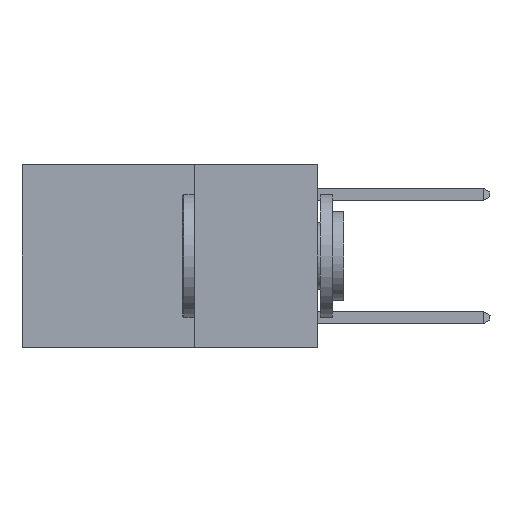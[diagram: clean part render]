
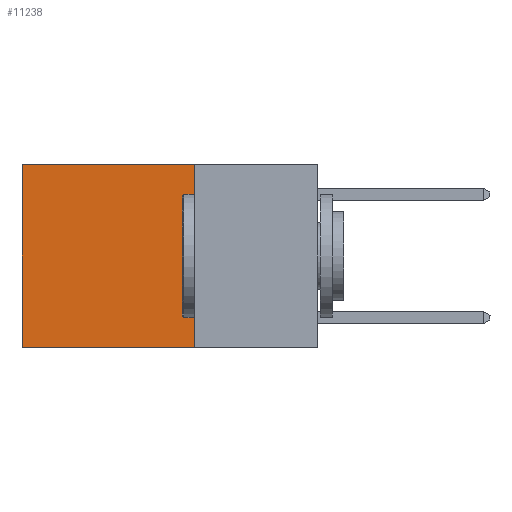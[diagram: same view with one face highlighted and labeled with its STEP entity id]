
A CAD part, left-side view. The second image highlights one B-rep face of the part: STEP entity #11238.
In plain terms, the highlighted planar face has unit normal (-1, 0, 0).
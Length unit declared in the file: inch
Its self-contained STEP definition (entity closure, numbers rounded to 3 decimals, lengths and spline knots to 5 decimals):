
#74 = VERTEX_POINT ( 'NONE', #15910 ) ;
#91 = DIRECTION ( 'NONE',  ( 0., 0., -1. ) ) ;
#204 = EDGE_CURVE ( 'NONE', #748, #74, #12748, .T. ) ;
#748 = VERTEX_POINT ( 'NONE', #11471 ) ;
#1539 = LINE ( 'NONE', #1663, #9656 ) ;
#1663 = CARTESIAN_POINT ( 'NONE',  ( 0.2625, 0.6, 0. ) ) ;
#3444 = CARTESIAN_POINT ( 'NONE',  ( 0.2625, 0.25, 0. ) ) ;
#3740 = FACE_OUTER_BOUND ( 'NONE', #8065, .T. ) ;
#3972 = ORIENTED_EDGE ( 'NONE', *, *, #7504, .T. ) ;
#3977 = ORIENTED_EDGE ( 'NONE', *, *, #204, .T. ) ;
#4228 = VECTOR ( 'NONE', #9289, 39.37008 ) ;
#4678 = VECTOR ( 'NONE', #14865, 39.37008 ) ;
#4970 = EDGE_CURVE ( 'NONE', #9615, #19525, #13573, .T. ) ;
#5723 = VECTOR ( 'NONE', #91, 39.37008 ) ;
#6664 = CARTESIAN_POINT ( 'NONE',  ( 0.2625, 0.25, 0. ) ) ;
#7197 = LINE ( 'NONE', #6664, #5723 ) ;
#7504 = EDGE_CURVE ( 'NONE', #74, #19525, #1539, .T. ) ;
#7704 = CARTESIAN_POINT ( 'NONE',  ( 0.2625, 0.25, -0.37 ) ) ;
#7995 = CARTESIAN_POINT ( 'NONE',  ( 0.2625, 0.6, -0.37 ) ) ;
#8065 = EDGE_LOOP ( 'NONE', ( #3972, #15941, #16909, #3977 ) ) ;
#9289 = DIRECTION ( 'NONE',  ( 0., 1., 0. ) ) ;
#9615 = VERTEX_POINT ( 'NONE', #13500 ) ;
#9656 = VECTOR ( 'NONE', #12614, 39.37008 ) ;
#11238 = ADVANCED_FACE ( 'NONE', ( #3740 ), #19020, .F. ) ;
#11471 = CARTESIAN_POINT ( 'NONE',  ( 0.2625, 0.25, 0. ) ) ;
#12614 = DIRECTION ( 'NONE',  ( 0., 0., -1. ) ) ;
#12748 = LINE ( 'NONE', #13276, #4678 ) ;
#13276 = CARTESIAN_POINT ( 'NONE',  ( 0.2625, 0.25, 0. ) ) ;
#13500 = CARTESIAN_POINT ( 'NONE',  ( 0.2625, 0.25, -0.37 ) ) ;
#13573 = LINE ( 'NONE', #7704, #4228 ) ;
#14391 = DIRECTION ( 'NONE',  ( 1., 0., 0. ) ) ;
#14865 = DIRECTION ( 'NONE',  ( 0., 1., 0. ) ) ;
#15910 = CARTESIAN_POINT ( 'NONE',  ( 0.2625, 0.6, 0. ) ) ;
#15941 = ORIENTED_EDGE ( 'NONE', *, *, #4970, .F. ) ;
#16683 = AXIS2_PLACEMENT_3D ( 'NONE', #3444, #14391, #18053 ) ;
#16909 = ORIENTED_EDGE ( 'NONE', *, *, #18499, .F. ) ;
#18053 = DIRECTION ( 'NONE',  ( 0., 0., -1. ) ) ;
#18499 = EDGE_CURVE ( 'NONE', #748, #9615, #7197, .T. ) ;
#19020 = PLANE ( 'NONE',  #16683 ) ;
#19525 = VERTEX_POINT ( 'NONE', #7995 ) ;
